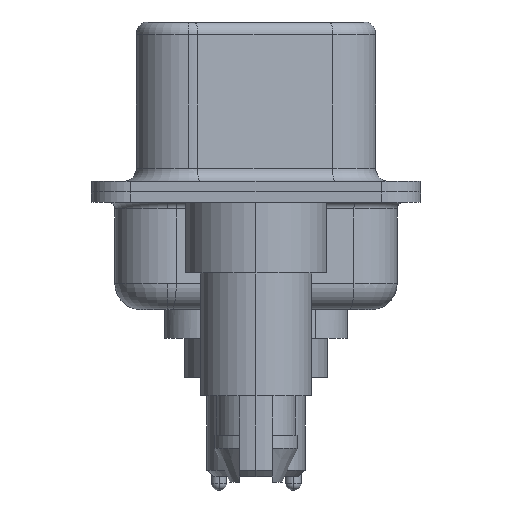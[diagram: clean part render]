
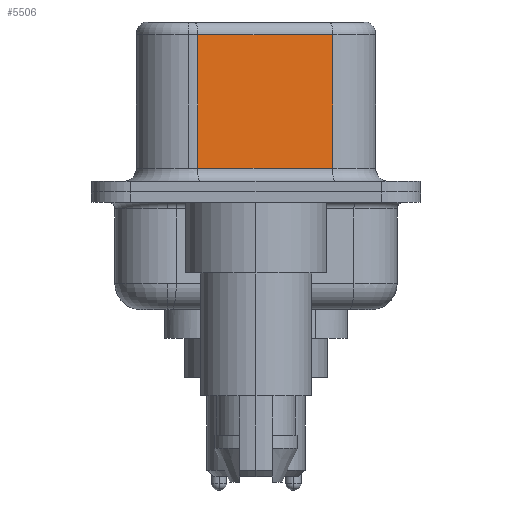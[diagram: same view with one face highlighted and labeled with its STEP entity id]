
A CAD part, left-side view. The second image highlights one B-rep face of the part: STEP entity #5506.
In plain terms, the highlighted planar face has unit normal (-0.985, -0.174, 0).
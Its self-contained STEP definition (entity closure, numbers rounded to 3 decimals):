
#221 = FACE_OUTER_BOUND ( 'NONE', #8554, .T. ) ;
#486 = CARTESIAN_POINT ( 'NONE',  ( 4.585, -2.927, 6.02 ) ) ;
#1686 = ORIENTED_EDGE ( 'NONE', *, *, #1766, .T. ) ;
#1707 = VECTOR ( 'NONE', #9308, 1000. ) ;
#1766 = EDGE_CURVE ( 'NONE', #10749, #8974, #2945, .T. ) ;
#2945 = LINE ( 'NONE', #3042, #13634 ) ;
#3042 = CARTESIAN_POINT ( 'NONE',  ( 3.675, 2.233, 6.52 ) ) ;
#4059 = EDGE_CURVE ( 'NONE', #8974, #8852, #11811, .T. ) ;
#4859 = CARTESIAN_POINT ( 'NONE',  ( 4.585, -2.927, 0.9 ) ) ;
#4972 = CARTESIAN_POINT ( 'NONE',  ( 3.675, 2.233, 6.02 ) ) ;
#4978 = LINE ( 'NONE', #486, #1707 ) ;
#5506 = ADVANCED_FACE ( 'NONE', ( #221 ), #15302, .F. ) ;
#6274 = CARTESIAN_POINT ( 'NONE',  ( 4.585, -2.927, 6.02 ) ) ;
#6631 = LINE ( 'NONE', #6846, #17287 ) ;
#6715 = CARTESIAN_POINT ( 'NONE',  ( 4.585, -2.927, 0.9 ) ) ;
#6823 = AXIS2_PLACEMENT_3D ( 'NONE', #16306, #16909, #14794 ) ;
#6846 = CARTESIAN_POINT ( 'NONE',  ( 4.585, -2.927, 6.52 ) ) ;
#7331 = EDGE_CURVE ( 'NONE', #13602, #10749, #4978, .T. ) ;
#8524 = ORIENTED_EDGE ( 'NONE', *, *, #4059, .T. ) ;
#8554 = EDGE_LOOP ( 'NONE', ( #16183, #9306, #1686, #8524 ) ) ;
#8852 = VERTEX_POINT ( 'NONE', #6715 ) ;
#8974 = VERTEX_POINT ( 'NONE', #13920 ) ;
#9306 = ORIENTED_EDGE ( 'NONE', *, *, #7331, .T. ) ;
#9308 = DIRECTION ( 'NONE',  ( -0.174, 0.985, 0. ) ) ;
#10749 = VERTEX_POINT ( 'NONE', #4972 ) ;
#11811 = LINE ( 'NONE', #4859, #15083 ) ;
#12537 = DIRECTION ( 'NONE',  ( 0.174, -0.985, 0. ) ) ;
#13602 = VERTEX_POINT ( 'NONE', #6274 ) ;
#13634 = VECTOR ( 'NONE', #16439, 1000. ) ;
#13920 = CARTESIAN_POINT ( 'NONE',  ( 3.675, 2.233, 0.9 ) ) ;
#14794 = DIRECTION ( 'NONE',  ( -0.174, 0.985, 0. ) ) ;
#15036 = EDGE_CURVE ( 'NONE', #13602, #8852, #6631, .T. ) ;
#15083 = VECTOR ( 'NONE', #12537, 1000. ) ;
#15196 = DIRECTION ( 'NONE',  ( 0., 0., -1. ) ) ;
#15302 = PLANE ( 'NONE',  #6823 ) ;
#16183 = ORIENTED_EDGE ( 'NONE', *, *, #15036, .F. ) ;
#16306 = CARTESIAN_POINT ( 'NONE',  ( 4.585, -2.927, 6.52 ) ) ;
#16439 = DIRECTION ( 'NONE',  ( 0., 0., -1. ) ) ;
#16909 = DIRECTION ( 'NONE',  ( 0.985, 0.174, 0. ) ) ;
#17287 = VECTOR ( 'NONE', #15196, 1000. ) ;
